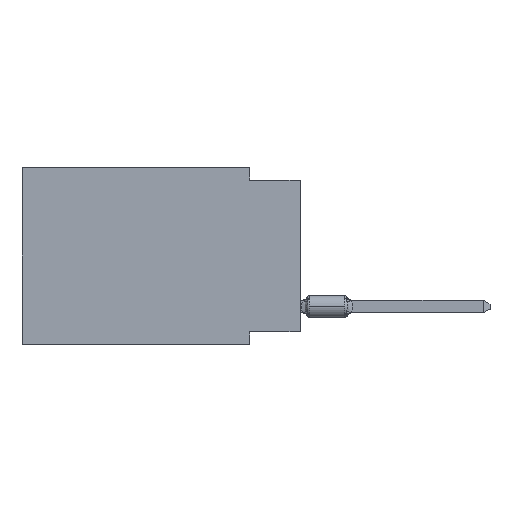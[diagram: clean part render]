
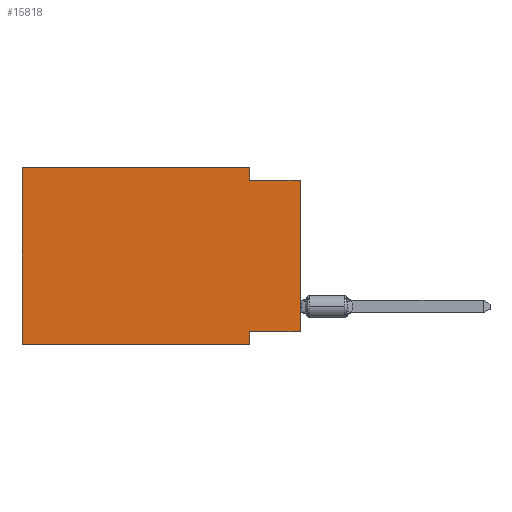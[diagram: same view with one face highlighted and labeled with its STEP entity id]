
A CAD part, left-side view. The second image highlights one B-rep face of the part: STEP entity #15818.
In plain terms, the highlighted planar face has unit normal (-1, 0, 0).
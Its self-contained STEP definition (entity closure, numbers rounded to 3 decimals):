
#36 = EDGE_CURVE ( 'NONE', #6496, #4201, #5665, .T. ) ;
#297 = CARTESIAN_POINT ( 'NONE',  ( 0., 2.54, 0. ) ) ;
#683 = CARTESIAN_POINT ( 'NONE',  ( 0., 13.97, 0. ) ) ;
#1003 = CARTESIAN_POINT ( 'NONE',  ( 0., 13.97, -8.89 ) ) ;
#1411 = CARTESIAN_POINT ( 'NONE',  ( 0., 13.97, 0. ) ) ;
#1704 = DIRECTION ( 'NONE',  ( 0., 1., 0. ) ) ;
#2000 = VERTEX_POINT ( 'NONE', #11504 ) ;
#2884 = DIRECTION ( 'NONE',  ( 0., 0., 1. ) ) ;
#3271 = ORIENTED_EDGE ( 'NONE', *, *, #16660, .F. ) ;
#3452 = CARTESIAN_POINT ( 'NONE',  ( 0., 0., -0.635 ) ) ;
#3734 = VERTEX_POINT ( 'NONE', #12267 ) ;
#3825 = CARTESIAN_POINT ( 'NONE',  ( 0., 0., 0. ) ) ;
#4000 = EDGE_LOOP ( 'NONE', ( #10140, #16895, #18245, #10611, #18934, #9150, #18723, #3271 ) ) ;
#4201 = VERTEX_POINT ( 'NONE', #14549 ) ;
#4583 = VECTOR ( 'NONE', #2884, 1000. ) ;
#4708 = EDGE_CURVE ( 'NONE', #15800, #6496, #19322, .T. ) ;
#4883 = CARTESIAN_POINT ( 'NONE',  ( 0., 13.97, 0. ) ) ;
#5201 = VECTOR ( 'NONE', #6974, 1000. ) ;
#5665 = LINE ( 'NONE', #11638, #16439 ) ;
#6294 = CARTESIAN_POINT ( 'NONE',  ( 0., 2.54, -8.255 ) ) ;
#6496 = VERTEX_POINT ( 'NONE', #683 ) ;
#6632 = FACE_OUTER_BOUND ( 'NONE', #4000, .T. ) ;
#6706 = CARTESIAN_POINT ( 'NONE',  ( 0., 0., -8.255 ) ) ;
#6762 = LINE ( 'NONE', #3825, #17942 ) ;
#6794 = VERTEX_POINT ( 'NONE', #10651 ) ;
#6974 = DIRECTION ( 'NONE',  ( 0., -1., 0. ) ) ;
#7454 = CARTESIAN_POINT ( 'NONE',  ( 0., 2.54, -8.89 ) ) ;
#8759 = VERTEX_POINT ( 'NONE', #6706 ) ;
#9148 = LINE ( 'NONE', #15120, #14896 ) ;
#9150 = ORIENTED_EDGE ( 'NONE', *, *, #16795, .T. ) ;
#9360 = EDGE_CURVE ( 'NONE', #14956, #3734, #10387, .T. ) ;
#10140 = ORIENTED_EDGE ( 'NONE', *, *, #18355, .T. ) ;
#10387 = LINE ( 'NONE', #7454, #13588 ) ;
#10500 = DIRECTION ( 'NONE',  ( 0., -1., 0. ) ) ;
#10611 = ORIENTED_EDGE ( 'NONE', *, *, #36, .F. ) ;
#10651 = CARTESIAN_POINT ( 'NONE',  ( 0., 2.54, -0.635 ) ) ;
#10854 = DIRECTION ( 'NONE',  ( 1., 0., 0. ) ) ;
#11504 = CARTESIAN_POINT ( 'NONE',  ( 0., 0., -0.635 ) ) ;
#11638 = CARTESIAN_POINT ( 'NONE',  ( 0., 13.97, 0. ) ) ;
#12012 = EDGE_CURVE ( 'NONE', #6794, #2000, #15003, .T. ) ;
#12267 = CARTESIAN_POINT ( 'NONE',  ( 0., 2.54, -8.89 ) ) ;
#12312 = CARTESIAN_POINT ( 'NONE',  ( 0., 13.97, -8.89 ) ) ;
#13588 = VECTOR ( 'NONE', #15184, 1000. ) ;
#13594 = EDGE_CURVE ( 'NONE', #4201, #6794, #18293, .T. ) ;
#14065 = DIRECTION ( 'NONE',  ( 0., 0., -1. ) ) ;
#14415 = LINE ( 'NONE', #1003, #5201 ) ;
#14549 = CARTESIAN_POINT ( 'NONE',  ( 0., 2.54, 0. ) ) ;
#14896 = VECTOR ( 'NONE', #1704, 1000. ) ;
#14956 = VERTEX_POINT ( 'NONE', #6294 ) ;
#15003 = LINE ( 'NONE', #3452, #15998 ) ;
#15120 = CARTESIAN_POINT ( 'NONE',  ( 0., 0., -8.255 ) ) ;
#15184 = DIRECTION ( 'NONE',  ( 0., 0., -1. ) ) ;
#15543 = PLANE ( 'NONE',  #17718 ) ;
#15800 = VERTEX_POINT ( 'NONE', #12312 ) ;
#15818 = ADVANCED_FACE ( 'NONE', ( #6632 ), #15543, .F. ) ;
#15998 = VECTOR ( 'NONE', #10500, 1000. ) ;
#16439 = VECTOR ( 'NONE', #17596, 1000. ) ;
#16660 = EDGE_CURVE ( 'NONE', #8759, #14956, #9148, .T. ) ;
#16795 = EDGE_CURVE ( 'NONE', #15800, #3734, #14415, .T. ) ;
#16895 = ORIENTED_EDGE ( 'NONE', *, *, #12012, .F. ) ;
#17596 = DIRECTION ( 'NONE',  ( 0., -1., 0. ) ) ;
#17718 = AXIS2_PLACEMENT_3D ( 'NONE', #4883, #10854, #14065 ) ;
#17942 = VECTOR ( 'NONE', #18597, 1000. ) ;
#18105 = DIRECTION ( 'NONE',  ( 0., 0., -1. ) ) ;
#18245 = ORIENTED_EDGE ( 'NONE', *, *, #13594, .F. ) ;
#18293 = LINE ( 'NONE', #297, #19097 ) ;
#18355 = EDGE_CURVE ( 'NONE', #8759, #2000, #6762, .T. ) ;
#18597 = DIRECTION ( 'NONE',  ( 0., 0., 1. ) ) ;
#18723 = ORIENTED_EDGE ( 'NONE', *, *, #9360, .F. ) ;
#18934 = ORIENTED_EDGE ( 'NONE', *, *, #4708, .F. ) ;
#19097 = VECTOR ( 'NONE', #18105, 1000. ) ;
#19322 = LINE ( 'NONE', #1411, #4583 ) ;
